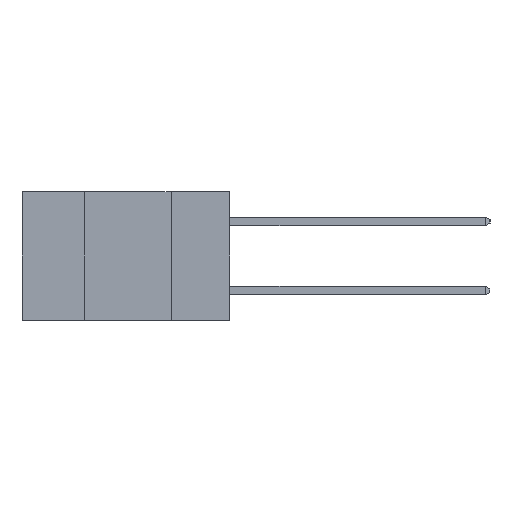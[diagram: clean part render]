
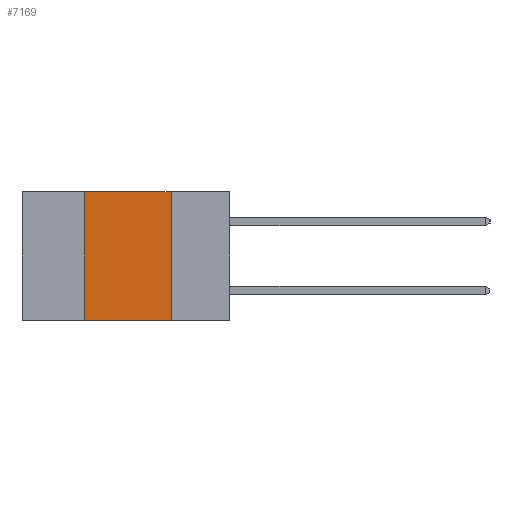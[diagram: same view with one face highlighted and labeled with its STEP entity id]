
A CAD part, left-side view. The second image highlights one B-rep face of the part: STEP entity #7169.
In plain terms, the highlighted planar face has unit normal (-1, 0, 0).
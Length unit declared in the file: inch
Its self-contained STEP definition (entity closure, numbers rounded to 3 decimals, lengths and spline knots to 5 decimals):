
#147 = ORIENTED_EDGE ( 'NONE', *, *, #777, .F. ) ;
#376 = DIRECTION ( 'NONE',  ( 0., 0., 1. ) ) ;
#680 = DIRECTION ( 'NONE',  ( 1., 0., 0. ) ) ;
#777 = EDGE_CURVE ( 'NONE', #11600, #11018, #9401, .T. ) ;
#1288 = VERTEX_POINT ( 'NONE', #2504 ) ;
#1485 = CARTESIAN_POINT ( 'NONE',  ( 0., 0.42, 0. ) ) ;
#1551 = ORIENTED_EDGE ( 'NONE', *, *, #8949, .F. ) ;
#2262 = VECTOR ( 'NONE', #6289, 39.37008 ) ;
#2369 = EDGE_CURVE ( 'NONE', #1288, #5415, #6299, .T. ) ;
#2405 = CARTESIAN_POINT ( 'NONE',  ( 0., 0.17, 0. ) ) ;
#2504 = CARTESIAN_POINT ( 'NONE',  ( 0., 0.42, -0.37 ) ) ;
#2612 = EDGE_LOOP ( 'NONE', ( #147, #1551, #6461, #11199 ) ) ;
#2804 = CARTESIAN_POINT ( 'NONE',  ( 0., 0.17, 0. ) ) ;
#3234 = EDGE_CURVE ( 'NONE', #1288, #11018, #11830, .T. ) ;
#3323 = CARTESIAN_POINT ( 'NONE',  ( 0., 0.17, -0.37 ) ) ;
#3871 = VECTOR ( 'NONE', #376, 39.37008 ) ;
#4621 = VECTOR ( 'NONE', #11631, 39.37008 ) ;
#5160 = DIRECTION ( 'NONE',  ( 0., -1., 0. ) ) ;
#5365 = CARTESIAN_POINT ( 'NONE',  ( 0., 0.6, 0. ) ) ;
#5415 = VERTEX_POINT ( 'NONE', #11378 ) ;
#6289 = DIRECTION ( 'NONE',  ( 0., -1., 0. ) ) ;
#6299 = LINE ( 'NONE', #1485, #3871 ) ;
#6461 = ORIENTED_EDGE ( 'NONE', *, *, #2369, .F. ) ;
#7140 = DIRECTION ( 'NONE',  ( 0., 0., -1. ) ) ;
#7169 = ADVANCED_FACE ( 'NONE', ( #10261 ), #8026, .F. ) ;
#8026 = PLANE ( 'NONE',  #8585 ) ;
#8376 = VECTOR ( 'NONE', #5160, 39.37008 ) ;
#8585 = AXIS2_PLACEMENT_3D ( 'NONE', #5365, #680, #7140 ) ;
#8942 = LINE ( 'NONE', #10500, #8376 ) ;
#8949 = EDGE_CURVE ( 'NONE', #5415, #11600, #8942, .T. ) ;
#9401 = LINE ( 'NONE', #2804, #4621 ) ;
#9720 = CARTESIAN_POINT ( 'NONE',  ( 0., 0.6, -0.37 ) ) ;
#10261 = FACE_OUTER_BOUND ( 'NONE', #2612, .T. ) ;
#10500 = CARTESIAN_POINT ( 'NONE',  ( 0., 0.6, 0. ) ) ;
#11018 = VERTEX_POINT ( 'NONE', #3323 ) ;
#11199 = ORIENTED_EDGE ( 'NONE', *, *, #3234, .T. ) ;
#11378 = CARTESIAN_POINT ( 'NONE',  ( 0., 0.42, 0. ) ) ;
#11600 = VERTEX_POINT ( 'NONE', #2405 ) ;
#11631 = DIRECTION ( 'NONE',  ( 0., 0., -1. ) ) ;
#11830 = LINE ( 'NONE', #9720, #2262 ) ;
